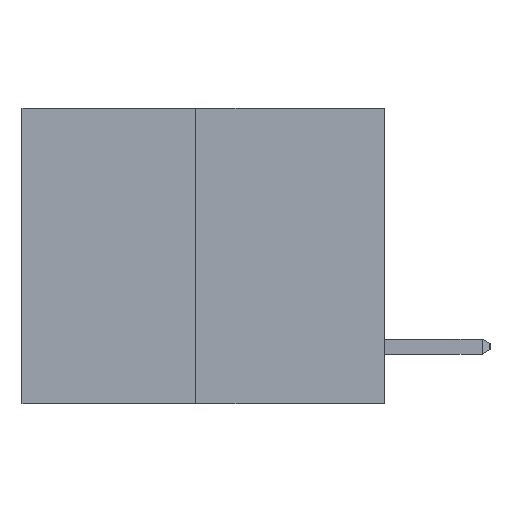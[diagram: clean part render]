
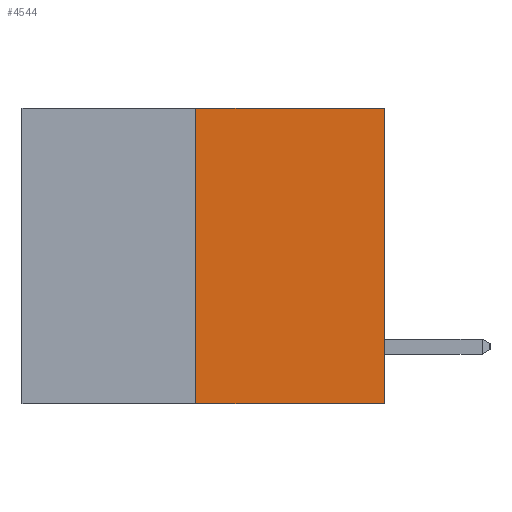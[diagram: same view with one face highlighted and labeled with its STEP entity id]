
A CAD part, left-side view. The second image highlights one B-rep face of the part: STEP entity #4544.
In plain terms, the highlighted planar face has unit normal (-1, 0, 0).
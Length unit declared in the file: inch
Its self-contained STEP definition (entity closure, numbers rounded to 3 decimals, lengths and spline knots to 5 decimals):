
#299 = ORIENTED_EDGE ( 'NONE', *, *, #10652, .T. ) ;
#620 = ORIENTED_EDGE ( 'NONE', *, *, #5114, .T. ) ;
#795 = LINE ( 'NONE', #2429, #10641 ) ;
#1087 = DIRECTION ( 'NONE',  ( 0., 0., 1. ) ) ;
#1904 = CARTESIAN_POINT ( 'NONE',  ( 0., 0.312, -0.49 ) ) ;
#2145 = ORIENTED_EDGE ( 'NONE', *, *, #11850, .F. ) ;
#2429 = CARTESIAN_POINT ( 'NONE',  ( 0., 0.6, 0. ) ) ;
#2557 = CARTESIAN_POINT ( 'NONE',  ( 0., 0., -0.49 ) ) ;
#3485 = DIRECTION ( 'NONE',  ( 0., 0., 1. ) ) ;
#3539 = CARTESIAN_POINT ( 'NONE',  ( 0., 0.312, -0.49 ) ) ;
#3660 = VERTEX_POINT ( 'NONE', #1904 ) ;
#4021 = AXIS2_PLACEMENT_3D ( 'NONE', #10354, #6825, #5666 ) ;
#4378 = VECTOR ( 'NONE', #1087, 39.37008 ) ;
#4544 = ADVANCED_FACE ( 'NONE', ( #6841 ), #13793, .F. ) ;
#4698 = LINE ( 'NONE', #11730, #6148 ) ;
#5114 = EDGE_CURVE ( 'NONE', #3660, #14154, #4698, .T. ) ;
#5501 = VECTOR ( 'NONE', #3485, 39.37008 ) ;
#5591 = VERTEX_POINT ( 'NONE', #14634 ) ;
#5666 = DIRECTION ( 'NONE',  ( 0., 0., -1. ) ) ;
#5692 = EDGE_CURVE ( 'NONE', #8423, #5591, #795, .T. ) ;
#6148 = VECTOR ( 'NONE', #7159, 39.37008 ) ;
#6825 = DIRECTION ( 'NONE',  ( 1., 0., 0. ) ) ;
#6841 = FACE_OUTER_BOUND ( 'NONE', #9156, .T. ) ;
#7159 = DIRECTION ( 'NONE',  ( 0., -1., 0. ) ) ;
#8423 = VERTEX_POINT ( 'NONE', #12377 ) ;
#9156 = EDGE_LOOP ( 'NONE', ( #2145, #620, #299, #13257 ) ) ;
#10354 = CARTESIAN_POINT ( 'NONE',  ( 0., 0.6, 0. ) ) ;
#10641 = VECTOR ( 'NONE', #12801, 39.37008 ) ;
#10652 = EDGE_CURVE ( 'NONE', #14154, #5591, #11733, .T. ) ;
#11730 = CARTESIAN_POINT ( 'NONE',  ( 0., 0.6, -0.49 ) ) ;
#11733 = LINE ( 'NONE', #13817, #4378 ) ;
#11850 = EDGE_CURVE ( 'NONE', #3660, #8423, #13991, .T. ) ;
#12377 = CARTESIAN_POINT ( 'NONE',  ( 0., 0.312, 0. ) ) ;
#12801 = DIRECTION ( 'NONE',  ( 0., -1., 0. ) ) ;
#13257 = ORIENTED_EDGE ( 'NONE', *, *, #5692, .F. ) ;
#13793 = PLANE ( 'NONE',  #4021 ) ;
#13817 = CARTESIAN_POINT ( 'NONE',  ( 0., 0., 0. ) ) ;
#13991 = LINE ( 'NONE', #3539, #5501 ) ;
#14154 = VERTEX_POINT ( 'NONE', #2557 ) ;
#14634 = CARTESIAN_POINT ( 'NONE',  ( 0., 0., 0. ) ) ;
